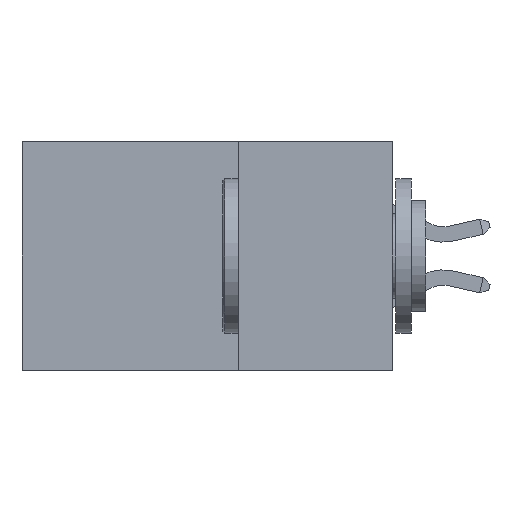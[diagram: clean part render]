
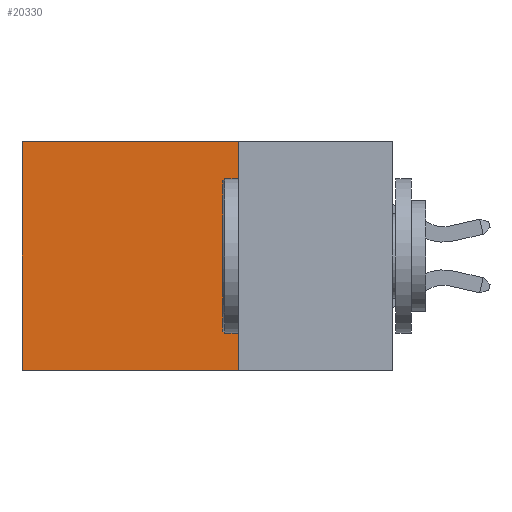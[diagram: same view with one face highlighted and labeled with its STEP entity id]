
A CAD part, left-side view. The second image highlights one B-rep face of the part: STEP entity #20330.
In plain terms, the highlighted planar face has unit normal (-1, 0, 0).
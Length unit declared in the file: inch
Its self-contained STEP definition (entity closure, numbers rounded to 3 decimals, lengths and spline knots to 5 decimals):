
#131 = DIRECTION ( 'NONE',  ( 1., 0., 0. ) ) ;
#262 = CARTESIAN_POINT ( 'NONE',  ( 0.2875, 0.25, 0. ) ) ;
#659 = CARTESIAN_POINT ( 'NONE',  ( 0.2875, 0.25, 0. ) ) ;
#912 = ORIENTED_EDGE ( 'NONE', *, *, #8617, .T. ) ;
#1482 = DIRECTION ( 'NONE',  ( 0., 1., 0. ) ) ;
#2399 = ORIENTED_EDGE ( 'NONE', *, *, #4075, .T. ) ;
#4075 = EDGE_CURVE ( 'NONE', #26604, #24971, #26372, .T. ) ;
#4434 = VECTOR ( 'NONE', #16932, 39.37008 ) ;
#4863 = CARTESIAN_POINT ( 'NONE',  ( 0.2875, 0.6, 0. ) ) ;
#6834 = PLANE ( 'NONE',  #30910 ) ;
#6939 = ORIENTED_EDGE ( 'NONE', *, *, #20435, .F. ) ;
#8617 = EDGE_CURVE ( 'NONE', #24971, #32772, #23917, .T. ) ;
#9995 = LINE ( 'NONE', #21027, #13534 ) ;
#10343 = VERTEX_POINT ( 'NONE', #25637 ) ;
#13221 = EDGE_LOOP ( 'NONE', ( #912, #15289, #6939, #2399 ) ) ;
#13534 = VECTOR ( 'NONE', #1482, 39.37008 ) ;
#13815 = CARTESIAN_POINT ( 'NONE',  ( 0.2875, 0.25, 0. ) ) ;
#13939 = CARTESIAN_POINT ( 'NONE',  ( 0.2875, 0.25, 0. ) ) ;
#15289 = ORIENTED_EDGE ( 'NONE', *, *, #17002, .F. ) ;
#16630 = VECTOR ( 'NONE', #36564, 39.37008 ) ;
#16637 = LINE ( 'NONE', #13939, #4434 ) ;
#16932 = DIRECTION ( 'NONE',  ( 0., 0., -1. ) ) ;
#17002 = EDGE_CURVE ( 'NONE', #10343, #32772, #9995, .T. ) ;
#19331 = VECTOR ( 'NONE', #31000, 39.37008 ) ;
#20330 = ADVANCED_FACE ( 'NONE', ( #24848 ), #6834, .F. ) ;
#20435 = EDGE_CURVE ( 'NONE', #26604, #10343, #16637, .T. ) ;
#21027 = CARTESIAN_POINT ( 'NONE',  ( 0.2875, 0.25, -0.37 ) ) ;
#21469 = CARTESIAN_POINT ( 'NONE',  ( 0.2875, 0.6, 0. ) ) ;
#23096 = DIRECTION ( 'NONE',  ( 0., 0., -1. ) ) ;
#23917 = LINE ( 'NONE', #4863, #19331 ) ;
#24848 = FACE_OUTER_BOUND ( 'NONE', #13221, .T. ) ;
#24971 = VERTEX_POINT ( 'NONE', #21469 ) ;
#25637 = CARTESIAN_POINT ( 'NONE',  ( 0.2875, 0.25, -0.37 ) ) ;
#26372 = LINE ( 'NONE', #13815, #16630 ) ;
#26604 = VERTEX_POINT ( 'NONE', #659 ) ;
#28128 = CARTESIAN_POINT ( 'NONE',  ( 0.2875, 0.6, -0.37 ) ) ;
#30910 = AXIS2_PLACEMENT_3D ( 'NONE', #262, #131, #23096 ) ;
#31000 = DIRECTION ( 'NONE',  ( 0., 0., -1. ) ) ;
#32772 = VERTEX_POINT ( 'NONE', #28128 ) ;
#36564 = DIRECTION ( 'NONE',  ( 0., 1., 0. ) ) ;
